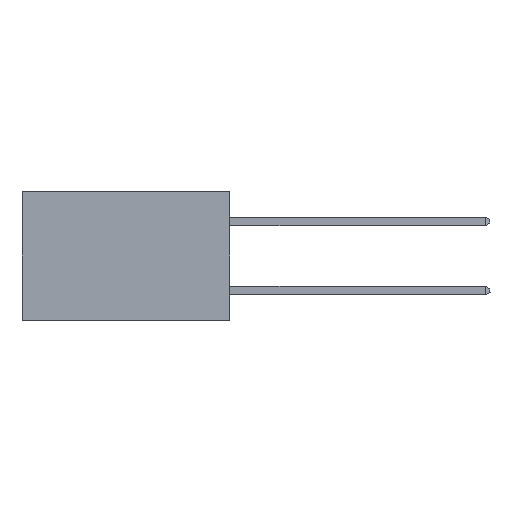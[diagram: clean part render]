
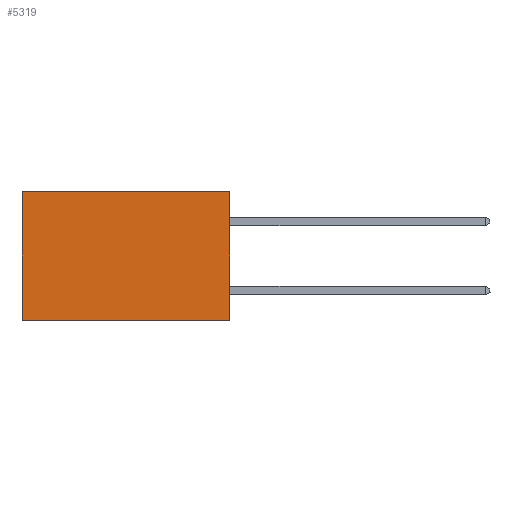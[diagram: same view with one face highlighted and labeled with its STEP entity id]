
A CAD part, left-side view. The second image highlights one B-rep face of the part: STEP entity #5319.
In plain terms, the highlighted planar face has unit normal (-1, 0, 0).
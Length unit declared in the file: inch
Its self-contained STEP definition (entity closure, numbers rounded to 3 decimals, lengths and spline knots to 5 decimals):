
#530 = VERTEX_POINT ( 'NONE', #6035 ) ;
#982 = LINE ( 'NONE', #14325, #2749 ) ;
#1891 = VECTOR ( 'NONE', #11603, 39.37008 ) ;
#2526 = EDGE_CURVE ( 'NONE', #4925, #8295, #982, .T. ) ;
#2749 = VECTOR ( 'NONE', #8617, 39.37008 ) ;
#3090 = EDGE_CURVE ( 'NONE', #4925, #13410, #5873, .T. ) ;
#3174 = CARTESIAN_POINT ( 'NONE',  ( 0.298, 0.6, 0. ) ) ;
#3928 = ORIENTED_EDGE ( 'NONE', *, *, #2526, .F. ) ;
#3940 = ORIENTED_EDGE ( 'NONE', *, *, #8343, .F. ) ;
#4262 = EDGE_CURVE ( 'NONE', #13410, #530, #7761, .T. ) ;
#4925 = VERTEX_POINT ( 'NONE', #10262 ) ;
#4991 = CARTESIAN_POINT ( 'NONE',  ( 0.298, 0., -0.37 ) ) ;
#5270 = FACE_OUTER_BOUND ( 'NONE', #6190, .T. ) ;
#5319 = ADVANCED_FACE ( 'NONE', ( #5270 ), #7078, .F. ) ;
#5394 = AXIS2_PLACEMENT_3D ( 'NONE', #8158, #5962, #11533 ) ;
#5730 = CARTESIAN_POINT ( 'NONE',  ( 0.298, 0., 0. ) ) ;
#5864 = CARTESIAN_POINT ( 'NONE',  ( 0.298, 0., -0.37 ) ) ;
#5873 = LINE ( 'NONE', #5730, #9033 ) ;
#5962 = DIRECTION ( 'NONE',  ( 1., 0., 0. ) ) ;
#6035 = CARTESIAN_POINT ( 'NONE',  ( 0.298, 0.6, -0.37 ) ) ;
#6190 = EDGE_LOOP ( 'NONE', ( #7248, #3940, #3928, #8823 ) ) ;
#7078 = PLANE ( 'NONE',  #5394 ) ;
#7147 = LINE ( 'NONE', #4991, #1891 ) ;
#7248 = ORIENTED_EDGE ( 'NONE', *, *, #4262, .T. ) ;
#7761 = LINE ( 'NONE', #14315, #10032 ) ;
#8158 = CARTESIAN_POINT ( 'NONE',  ( 0.298, 0., 0. ) ) ;
#8295 = VERTEX_POINT ( 'NONE', #5864 ) ;
#8343 = EDGE_CURVE ( 'NONE', #8295, #530, #7147, .T. ) ;
#8617 = DIRECTION ( 'NONE',  ( 0., 0., -1. ) ) ;
#8823 = ORIENTED_EDGE ( 'NONE', *, *, #3090, .T. ) ;
#9033 = VECTOR ( 'NONE', #9087, 39.37008 ) ;
#9087 = DIRECTION ( 'NONE',  ( 0., 1., 0. ) ) ;
#10032 = VECTOR ( 'NONE', #14551, 39.37008 ) ;
#10262 = CARTESIAN_POINT ( 'NONE',  ( 0.298, 0., 0. ) ) ;
#11533 = DIRECTION ( 'NONE',  ( 0., 0., -1. ) ) ;
#11603 = DIRECTION ( 'NONE',  ( 0., 1., 0. ) ) ;
#13410 = VERTEX_POINT ( 'NONE', #3174 ) ;
#14315 = CARTESIAN_POINT ( 'NONE',  ( 0.298, 0.6, 0. ) ) ;
#14325 = CARTESIAN_POINT ( 'NONE',  ( 0.298, 0., 0. ) ) ;
#14551 = DIRECTION ( 'NONE',  ( 0., 0., -1. ) ) ;
